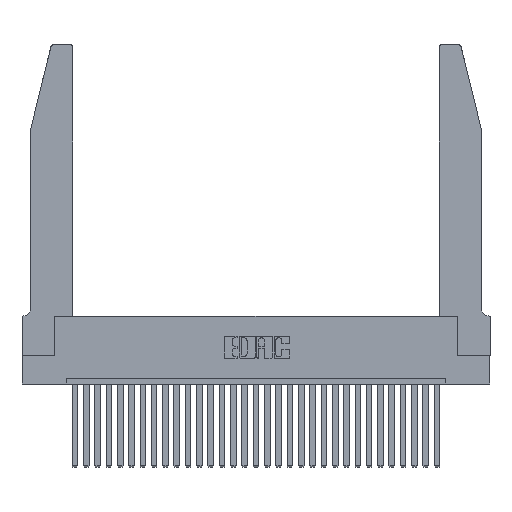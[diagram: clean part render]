
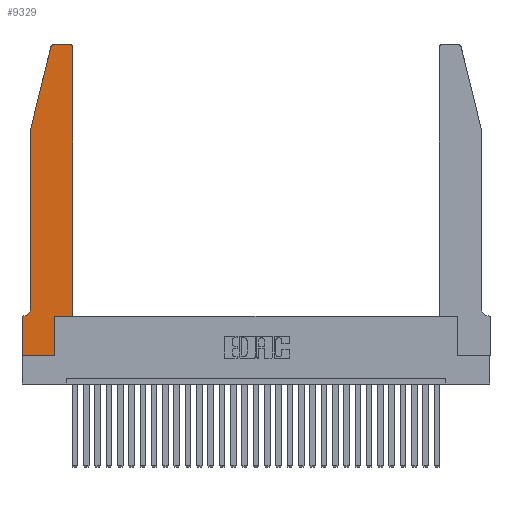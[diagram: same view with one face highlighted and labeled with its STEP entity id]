
A CAD part, top view. The second image highlights one B-rep face of the part: STEP entity #9329.
In plain terms, the highlighted planar face has unit normal (0, 0, 1).
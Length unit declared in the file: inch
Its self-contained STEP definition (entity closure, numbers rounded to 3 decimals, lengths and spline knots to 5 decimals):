
#89 = EDGE_CURVE ( 'NONE', #27598, #24152, #14662, .T. ) ;
#452 = DIRECTION ( 'NONE',  ( -1., 0., 0. ) ) ;
#1720 = VERTEX_POINT ( 'NONE', #9562 ) ;
#2084 = CARTESIAN_POINT ( 'NONE',  ( 0.284, 2.75, 0.37 ) ) ;
#2180 = DIRECTION ( 'NONE',  ( 1., 0., 0. ) ) ;
#2483 = EDGE_CURVE ( 'NONE', #24152, #25073, #22686, .T. ) ;
#3428 = CARTESIAN_POINT ( 'NONE',  ( 0., 0.35, 0.37 ) ) ;
#3532 = LINE ( 'NONE', #22169, #20554 ) ;
#3760 = VERTEX_POINT ( 'NONE', #7260 ) ;
#3989 = LINE ( 'NONE', #21379, #5082 ) ;
#4291 = VERTEX_POINT ( 'NONE', #2084 ) ;
#4929 = LINE ( 'NONE', #27320, #12701 ) ;
#5082 = VECTOR ( 'NONE', #452, 39.37008 ) ;
#5150 = CARTESIAN_POINT ( 'NONE',  ( 0., 0., 0.37 ) ) ;
#5911 = DIRECTION ( 'NONE',  ( 1., 0., 0. ) ) ;
#7260 = CARTESIAN_POINT ( 'NONE',  ( 0.2865, 0., 0.37 ) ) ;
#7266 = VECTOR ( 'NONE', #16909, 39.37008 ) ;
#7672 = CARTESIAN_POINT ( 'NONE',  ( 0.4505, 2.72, 0.37 ) ) ;
#8099 = ORIENTED_EDGE ( 'NONE', *, *, #2483, .T. ) ;
#8795 = CARTESIAN_POINT ( 'NONE',  ( 0.0055, 0.42, 0.37 ) ) ;
#9304 = CARTESIAN_POINT ( 'NONE',  ( 0.2605, 2.75, 0.37 ) ) ;
#9329 = ADVANCED_FACE ( 'NONE', ( #12160 ), #19649, .T. ) ;
#9425 = VECTOR ( 'NONE', #5911, 39.37008 ) ;
#9516 = AXIS2_PLACEMENT_3D ( 'NONE', #16337, #30646, #23474 ) ;
#9562 = CARTESIAN_POINT ( 'NONE',  ( 0.2865, 0.35, 0.37 ) ) ;
#9871 = VECTOR ( 'NONE', #24505, 39.37008 ) ;
#9976 = CARTESIAN_POINT ( 'NONE',  ( 0.0755, 0.42, 0.37 ) ) ;
#10352 = DIRECTION ( 'NONE',  ( 0., 0., 1. ) ) ;
#10554 = CARTESIAN_POINT ( 'NONE',  ( 0., 0., 0.37 ) ) ;
#10579 = EDGE_CURVE ( 'NONE', #28513, #13209, #29528, .T. ) ;
#10582 = CARTESIAN_POINT ( 'NONE',  ( 0., 0., 0.37 ) ) ;
#10626 = ORIENTED_EDGE ( 'NONE', *, *, #10579, .T. ) ;
#10917 = ORIENTED_EDGE ( 'NONE', *, *, #30291, .T. ) ;
#11175 = DIRECTION ( 'NONE',  ( -1., 0., 0. ) ) ;
#11405 = AXIS2_PLACEMENT_3D ( 'NONE', #3428, #10352, #26990 ) ;
#11533 = VECTOR ( 'NONE', #25882, 39.37008 ) ;
#12160 = FACE_OUTER_BOUND ( 'NONE', #26843, .T. ) ;
#12383 = EDGE_CURVE ( 'NONE', #1720, #27598, #26174, .T. ) ;
#12701 = VECTOR ( 'NONE', #20191, 39.37008 ) ;
#13209 = VERTEX_POINT ( 'NONE', #18322 ) ;
#13944 = CARTESIAN_POINT ( 'NONE',  ( 0.4205, 2.72, 0.37 ) ) ;
#14662 = LINE ( 'NONE', #24977, #28735 ) ;
#15310 = ORIENTED_EDGE ( 'NONE', *, *, #22578, .T. ) ;
#15691 = CARTESIAN_POINT ( 'NONE',  ( 0.4505, 0.35, 0.37 ) ) ;
#15799 = LINE ( 'NONE', #28594, #7266 ) ;
#15965 = DIRECTION ( 'NONE',  ( 1., 0., 0. ) ) ;
#16187 = LINE ( 'NONE', #5150, #9871 ) ;
#16337 = CARTESIAN_POINT ( 'NONE',  ( 0.284, 2.72, 0.37 ) ) ;
#16342 = DIRECTION ( 'NONE',  ( 0., 0., 1. ) ) ;
#16909 = DIRECTION ( 'NONE',  ( -0.239, -0.971, 0. ) ) ;
#16929 = ORIENTED_EDGE ( 'NONE', *, *, #28441, .T. ) ;
#17199 = EDGE_CURVE ( 'NONE', #3760, #1720, #4929, .T. ) ;
#17297 = ORIENTED_EDGE ( 'NONE', *, *, #89, .T. ) ;
#17567 = DIRECTION ( 'NONE',  ( 0., -1., 0. ) ) ;
#17767 = EDGE_CURVE ( 'NONE', #25073, #4291, #19312, .T. ) ;
#18322 = CARTESIAN_POINT ( 'NONE',  ( 0.0055, 0.35, 0.37 ) ) ;
#18771 = CARTESIAN_POINT ( 'NONE',  ( 0.0755, 2., 0.37 ) ) ;
#19006 = CARTESIAN_POINT ( 'NONE',  ( 0.4205, 2.75, 0.37 ) ) ;
#19061 = VERTEX_POINT ( 'NONE', #10582 ) ;
#19271 = VERTEX_POINT ( 'NONE', #29840 ) ;
#19312 = LINE ( 'NONE', #9304, #11533 ) ;
#19649 = PLANE ( 'NONE',  #11405 ) ;
#19678 = ORIENTED_EDGE ( 'NONE', *, *, #12383, .T. ) ;
#20191 = DIRECTION ( 'NONE',  ( 0., 1., 0. ) ) ;
#20554 = VECTOR ( 'NONE', #17567, 39.37008 ) ;
#20590 = DIRECTION ( 'NONE',  ( 0., 0., -1. ) ) ;
#20761 = AXIS2_PLACEMENT_3D ( 'NONE', #8795, #20590, #11175 ) ;
#21094 = CARTESIAN_POINT ( 'NONE',  ( 0.4505, 0.35, 0.37 ) ) ;
#21379 = CARTESIAN_POINT ( 'NONE',  ( 0.0755, 0.35, 0.37 ) ) ;
#21438 = EDGE_CURVE ( 'NONE', #4291, #19271, #26184, .T. ) ;
#21858 = ORIENTED_EDGE ( 'NONE', *, *, #17199, .T. ) ;
#22033 = LINE ( 'NONE', #10554, #9425 ) ;
#22169 = CARTESIAN_POINT ( 'NONE',  ( 0.0755, 2., 0.37 ) ) ;
#22486 = ORIENTED_EDGE ( 'NONE', *, *, #29463, .T. ) ;
#22578 = EDGE_CURVE ( 'NONE', #22917, #28513, #3532, .T. ) ;
#22686 = CIRCLE ( 'NONE', #27543, 0.03 ) ;
#22917 = VERTEX_POINT ( 'NONE', #18771 ) ;
#22942 = CARTESIAN_POINT ( 'NONE',  ( 0., 0.35, 0.37 ) ) ;
#23474 = DIRECTION ( 'NONE',  ( 1., 0., 0. ) ) ;
#23959 = VECTOR ( 'NONE', #15965, 39.37008 ) ;
#24152 = VERTEX_POINT ( 'NONE', #7672 ) ;
#24505 = DIRECTION ( 'NONE',  ( 0., -1., 0. ) ) ;
#24977 = CARTESIAN_POINT ( 'NONE',  ( 0.4505, 0.35, 0.37 ) ) ;
#25073 = VERTEX_POINT ( 'NONE', #19006 ) ;
#25882 = DIRECTION ( 'NONE',  ( -1., 0., 0. ) ) ;
#25959 = VERTEX_POINT ( 'NONE', #22942 ) ;
#26174 = LINE ( 'NONE', #21094, #23959 ) ;
#26184 = CIRCLE ( 'NONE', #9516, 0.03 ) ;
#26843 = EDGE_LOOP ( 'NONE', ( #30002, #30213, #10917, #15310, #10626, #16929, #28809, #22486, #21858, #19678, #17297, #8099 ) ) ;
#26990 = DIRECTION ( 'NONE',  ( 1., 0., 0. ) ) ;
#27320 = CARTESIAN_POINT ( 'NONE',  ( 0.2865, 0.35, 0.37 ) ) ;
#27443 = DIRECTION ( 'NONE',  ( 0., 1., 0. ) ) ;
#27543 = AXIS2_PLACEMENT_3D ( 'NONE', #13944, #16342, #2180 ) ;
#27598 = VERTEX_POINT ( 'NONE', #15691 ) ;
#28441 = EDGE_CURVE ( 'NONE', #13209, #25959, #3989, .T. ) ;
#28513 = VERTEX_POINT ( 'NONE', #9976 ) ;
#28594 = CARTESIAN_POINT ( 'NONE',  ( 0.0755, 2., 0.37 ) ) ;
#28735 = VECTOR ( 'NONE', #27443, 39.37008 ) ;
#28809 = ORIENTED_EDGE ( 'NONE', *, *, #29823, .T. ) ;
#29463 = EDGE_CURVE ( 'NONE', #19061, #3760, #22033, .T. ) ;
#29528 = CIRCLE ( 'NONE', #20761, 0.07 ) ;
#29823 = EDGE_CURVE ( 'NONE', #25959, #19061, #16187, .T. ) ;
#29840 = CARTESIAN_POINT ( 'NONE',  ( 0.25487, 2.72718, 0.37 ) ) ;
#30002 = ORIENTED_EDGE ( 'NONE', *, *, #17767, .T. ) ;
#30213 = ORIENTED_EDGE ( 'NONE', *, *, #21438, .T. ) ;
#30291 = EDGE_CURVE ( 'NONE', #19271, #22917, #15799, .T. ) ;
#30646 = DIRECTION ( 'NONE',  ( 0., 0., 1. ) ) ;
